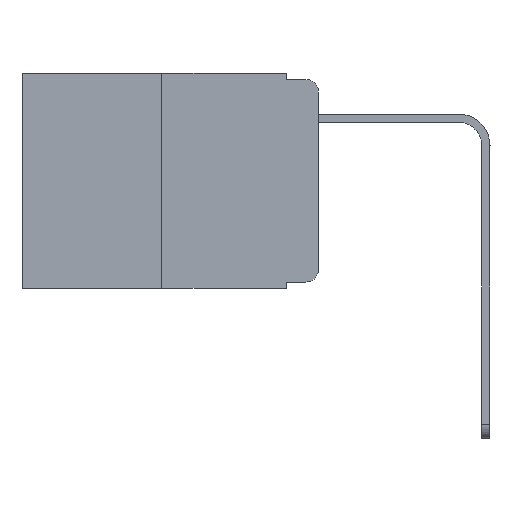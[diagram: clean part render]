
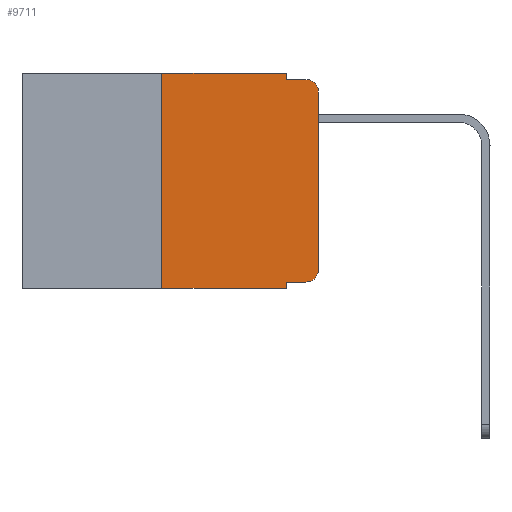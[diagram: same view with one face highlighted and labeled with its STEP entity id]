
A CAD part, left-side view. The second image highlights one B-rep face of the part: STEP entity #9711.
In plain terms, the highlighted planar face has unit normal (-1, 0, 0).
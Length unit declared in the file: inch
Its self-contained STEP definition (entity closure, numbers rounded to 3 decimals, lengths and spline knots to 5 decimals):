
#163 = VECTOR ( 'NONE', #8896, 39.37008 ) ;
#253 = ORIENTED_EDGE ( 'NONE', *, *, #6921, .F. ) ;
#451 = CIRCLE ( 'NONE', #9593, 0.02 ) ;
#514 = ORIENTED_EDGE ( 'NONE', *, *, #13821, .T. ) ;
#580 = LINE ( 'NONE', #2300, #163 ) ;
#825 = CARTESIAN_POINT ( 'NONE',  ( 0., 0.473, -0.343 ) ) ;
#1289 = VERTEX_POINT ( 'NONE', #13048 ) ;
#1909 = ORIENTED_EDGE ( 'NONE', *, *, #8819, .F. ) ;
#2013 = CARTESIAN_POINT ( 'NONE',  ( 0., 0.051, -0.333 ) ) ;
#2104 = ORIENTED_EDGE ( 'NONE', *, *, #2345, .F. ) ;
#2243 = CARTESIAN_POINT ( 'NONE',  ( 0., 0.02, -0.313 ) ) ;
#2300 = CARTESIAN_POINT ( 'NONE',  ( 0., 0.25, 0. ) ) ;
#2345 = EDGE_CURVE ( 'NONE', #14788, #1289, #9607, .T. ) ;
#2514 = DIRECTION ( 'NONE',  ( 1., 0., 0. ) ) ;
#2645 = LINE ( 'NONE', #7838, #10876 ) ;
#3111 = DIRECTION ( 'NONE',  ( -1., 0., 0. ) ) ;
#3223 = DIRECTION ( 'NONE',  ( 0., 0., -1. ) ) ;
#3273 = CARTESIAN_POINT ( 'NONE',  ( 0., 0.051, 0. ) ) ;
#3471 = VERTEX_POINT ( 'NONE', #8258 ) ;
#3670 = CARTESIAN_POINT ( 'NONE',  ( 0., 0.051, -0.01 ) ) ;
#3841 = PLANE ( 'NONE',  #12005 ) ;
#3907 = AXIS2_PLACEMENT_3D ( 'NONE', #13652, #3111, #3223 ) ;
#3953 = CARTESIAN_POINT ( 'NONE',  ( 0., 0.051, 0. ) ) ;
#4729 = EDGE_CURVE ( 'NONE', #11393, #1289, #8681, .T. ) ;
#4743 = VECTOR ( 'NONE', #6677, 39.37008 ) ;
#4989 = CARTESIAN_POINT ( 'NONE',  ( 0., 0.051, -0.343 ) ) ;
#5086 = CARTESIAN_POINT ( 'NONE',  ( 0., 0.051, 0. ) ) ;
#5481 = CARTESIAN_POINT ( 'NONE',  ( 0., 0., -0.03 ) ) ;
#5775 = ORIENTED_EDGE ( 'NONE', *, *, #4729, .T. ) ;
#5869 = EDGE_LOOP ( 'NONE', ( #514, #5775, #2104, #1909, #14797, #253, #13341, #16978, #12111, #16310 ) ) ;
#5915 = LINE ( 'NONE', #8173, #6933 ) ;
#6057 = DIRECTION ( 'NONE',  ( 0., 0., -1. ) ) ;
#6669 = VECTOR ( 'NONE', #6057, 39.37008 ) ;
#6677 = DIRECTION ( 'NONE',  ( 0., 0., -1. ) ) ;
#6921 = EDGE_CURVE ( 'NONE', #3471, #16669, #580, .T. ) ;
#6933 = VECTOR ( 'NONE', #10806, 39.37008 ) ;
#7162 = VECTOR ( 'NONE', #10977, 39.37008 ) ;
#7435 = CARTESIAN_POINT ( 'NONE',  ( 0., 0., -0.313 ) ) ;
#7838 = CARTESIAN_POINT ( 'NONE',  ( 0., 0.051, -0.333 ) ) ;
#8173 = CARTESIAN_POINT ( 'NONE',  ( 0., 0.473, 0. ) ) ;
#8258 = CARTESIAN_POINT ( 'NONE',  ( 0., 0.25, -0.343 ) ) ;
#8597 = VECTOR ( 'NONE', #14421, 39.37008 ) ;
#8681 = CIRCLE ( 'NONE', #3907, 0.02 ) ;
#8819 = EDGE_CURVE ( 'NONE', #9675, #14788, #9343, .T. ) ;
#8896 = DIRECTION ( 'NONE',  ( 0., 0., 1. ) ) ;
#9091 = EDGE_CURVE ( 'NONE', #3471, #11218, #14498, .T. ) ;
#9343 = LINE ( 'NONE', #3273, #6669 ) ;
#9593 = AXIS2_PLACEMENT_3D ( 'NONE', #2243, #13905, #15251 ) ;
#9607 = LINE ( 'NONE', #13020, #8597 ) ;
#9675 = VERTEX_POINT ( 'NONE', #5086 ) ;
#9711 = ADVANCED_FACE ( 'NONE', ( #16784 ), #3841, .F. ) ;
#10257 = LINE ( 'NONE', #13436, #7162 ) ;
#10665 = CARTESIAN_POINT ( 'NONE',  ( 0., 0.25, 0. ) ) ;
#10806 = DIRECTION ( 'NONE',  ( 0., -1., 0. ) ) ;
#10876 = VECTOR ( 'NONE', #14283, 39.37008 ) ;
#10977 = DIRECTION ( 'NONE',  ( 0., 0., 1. ) ) ;
#11067 = EDGE_CURVE ( 'NONE', #13862, #14142, #451, .T. ) ;
#11218 = VERTEX_POINT ( 'NONE', #4989 ) ;
#11393 = VERTEX_POINT ( 'NONE', #5481 ) ;
#11723 = LINE ( 'NONE', #3953, #4743 ) ;
#12005 = AXIS2_PLACEMENT_3D ( 'NONE', #13010, #2514, #15345 ) ;
#12111 = ORIENTED_EDGE ( 'NONE', *, *, #13548, .T. ) ;
#12300 = CARTESIAN_POINT ( 'NONE',  ( 0., 0.02, -0.333 ) ) ;
#12650 = DIRECTION ( 'NONE',  ( 0., -1., 0. ) ) ;
#13010 = CARTESIAN_POINT ( 'NONE',  ( 0., 0.473, 0. ) ) ;
#13020 = CARTESIAN_POINT ( 'NONE',  ( 0., 0.051, -0.01 ) ) ;
#13048 = CARTESIAN_POINT ( 'NONE',  ( 0., 0.02, -0.01 ) ) ;
#13341 = ORIENTED_EDGE ( 'NONE', *, *, #9091, .T. ) ;
#13436 = CARTESIAN_POINT ( 'NONE',  ( 0., 0., 0. ) ) ;
#13548 = EDGE_CURVE ( 'NONE', #13965, #13862, #2645, .T. ) ;
#13652 = CARTESIAN_POINT ( 'NONE',  ( 0., 0.02, -0.03 ) ) ;
#13821 = EDGE_CURVE ( 'NONE', #14142, #11393, #10257, .T. ) ;
#13862 = VERTEX_POINT ( 'NONE', #12300 ) ;
#13893 = EDGE_CURVE ( 'NONE', #16669, #9675, #5915, .T. ) ;
#13905 = DIRECTION ( 'NONE',  ( -1., 0., 0. ) ) ;
#13965 = VERTEX_POINT ( 'NONE', #2013 ) ;
#14142 = VERTEX_POINT ( 'NONE', #7435 ) ;
#14283 = DIRECTION ( 'NONE',  ( 0., -1., 0. ) ) ;
#14421 = DIRECTION ( 'NONE',  ( 0., -1., 0. ) ) ;
#14498 = LINE ( 'NONE', #825, #16338 ) ;
#14788 = VERTEX_POINT ( 'NONE', #3670 ) ;
#14797 = ORIENTED_EDGE ( 'NONE', *, *, #13893, .F. ) ;
#15251 = DIRECTION ( 'NONE',  ( 0., 0., -1. ) ) ;
#15345 = DIRECTION ( 'NONE',  ( 0., 0., -1. ) ) ;
#15825 = EDGE_CURVE ( 'NONE', #13965, #11218, #11723, .T. ) ;
#16310 = ORIENTED_EDGE ( 'NONE', *, *, #11067, .T. ) ;
#16338 = VECTOR ( 'NONE', #12650, 39.37008 ) ;
#16669 = VERTEX_POINT ( 'NONE', #10665 ) ;
#16784 = FACE_OUTER_BOUND ( 'NONE', #5869, .T. ) ;
#16978 = ORIENTED_EDGE ( 'NONE', *, *, #15825, .F. ) ;
